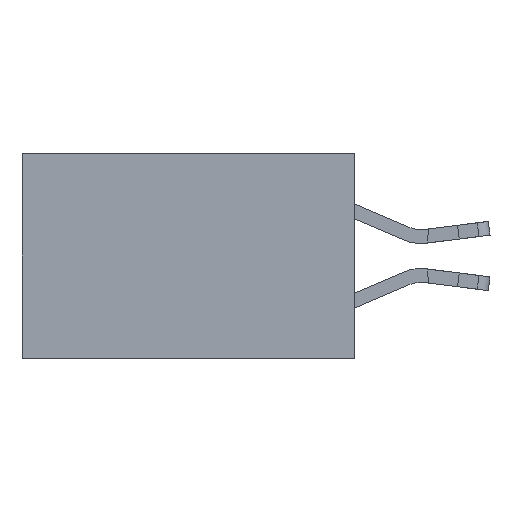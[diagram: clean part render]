
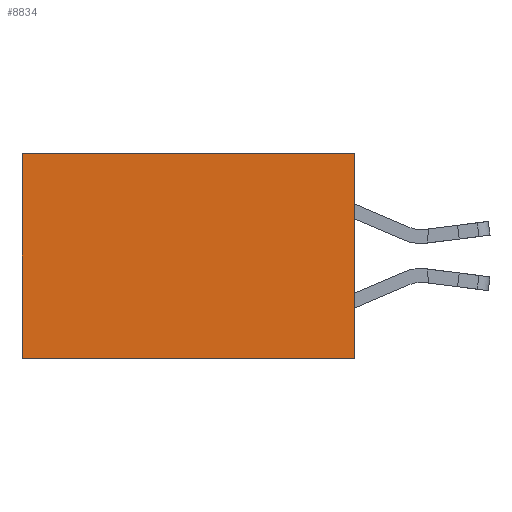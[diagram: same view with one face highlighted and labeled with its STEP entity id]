
A CAD part, left-side view. The second image highlights one B-rep face of the part: STEP entity #8834.
In plain terms, the highlighted planar face has unit normal (-1, 0, 0).
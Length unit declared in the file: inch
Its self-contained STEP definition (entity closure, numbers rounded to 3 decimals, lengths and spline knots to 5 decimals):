
#474 = VECTOR ( 'NONE', #21536, 39.37008 ) ;
#1003 = VERTEX_POINT ( 'NONE', #9414 ) ;
#1885 = LINE ( 'NONE', #7370, #13112 ) ;
#2134 = CARTESIAN_POINT ( 'NONE',  ( 0.298, 0., 0. ) ) ;
#2224 = VERTEX_POINT ( 'NONE', #9671 ) ;
#2751 = ORIENTED_EDGE ( 'NONE', *, *, #16308, .F. ) ;
#3227 = DIRECTION ( 'NONE',  ( 0., 1., 0. ) ) ;
#5758 = AXIS2_PLACEMENT_3D ( 'NONE', #2134, #24439, #11169 ) ;
#6031 = CARTESIAN_POINT ( 'NONE',  ( 0.298, 0.6, 0. ) ) ;
#6272 = DIRECTION ( 'NONE',  ( 0., 1., 0. ) ) ;
#6370 = ORIENTED_EDGE ( 'NONE', *, *, #18486, .T. ) ;
#6700 = PLANE ( 'NONE',  #5758 ) ;
#7370 = CARTESIAN_POINT ( 'NONE',  ( 0.298, 0., 0. ) ) ;
#8834 = ADVANCED_FACE ( 'NONE', ( #27793 ), #6700, .F. ) ;
#9414 = CARTESIAN_POINT ( 'NONE',  ( 0.298, 0., -0.37 ) ) ;
#9671 = CARTESIAN_POINT ( 'NONE',  ( 0.298, 0., 0. ) ) ;
#10651 = VECTOR ( 'NONE', #6272, 39.37008 ) ;
#11169 = DIRECTION ( 'NONE',  ( 0., 0., -1. ) ) ;
#12583 = ORIENTED_EDGE ( 'NONE', *, *, #26358, .T. ) ;
#13112 = VECTOR ( 'NONE', #20580, 39.37008 ) ;
#15332 = CARTESIAN_POINT ( 'NONE',  ( 0.298, 0.6, -0.37 ) ) ;
#15648 = EDGE_LOOP ( 'NONE', ( #6370, #2751, #19375, #12583 ) ) ;
#16308 = EDGE_CURVE ( 'NONE', #1003, #27096, #18729, .T. ) ;
#17323 = CARTESIAN_POINT ( 'NONE',  ( 0.298, 0., 0. ) ) ;
#18293 = LINE ( 'NONE', #6031, #474 ) ;
#18486 = EDGE_CURVE ( 'NONE', #27561, #27096, #18293, .T. ) ;
#18729 = LINE ( 'NONE', #27613, #23930 ) ;
#18953 = CARTESIAN_POINT ( 'NONE',  ( 0.298, 0.6, 0. ) ) ;
#19375 = ORIENTED_EDGE ( 'NONE', *, *, #25994, .F. ) ;
#20580 = DIRECTION ( 'NONE',  ( 0., 0., -1. ) ) ;
#21021 = LINE ( 'NONE', #17323, #10651 ) ;
#21536 = DIRECTION ( 'NONE',  ( 0., 0., -1. ) ) ;
#23930 = VECTOR ( 'NONE', #3227, 39.37008 ) ;
#24439 = DIRECTION ( 'NONE',  ( 1., 0., 0. ) ) ;
#25994 = EDGE_CURVE ( 'NONE', #2224, #1003, #1885, .T. ) ;
#26358 = EDGE_CURVE ( 'NONE', #2224, #27561, #21021, .T. ) ;
#27096 = VERTEX_POINT ( 'NONE', #15332 ) ;
#27561 = VERTEX_POINT ( 'NONE', #18953 ) ;
#27613 = CARTESIAN_POINT ( 'NONE',  ( 0.298, 0., -0.37 ) ) ;
#27793 = FACE_OUTER_BOUND ( 'NONE', #15648, .T. ) ;
